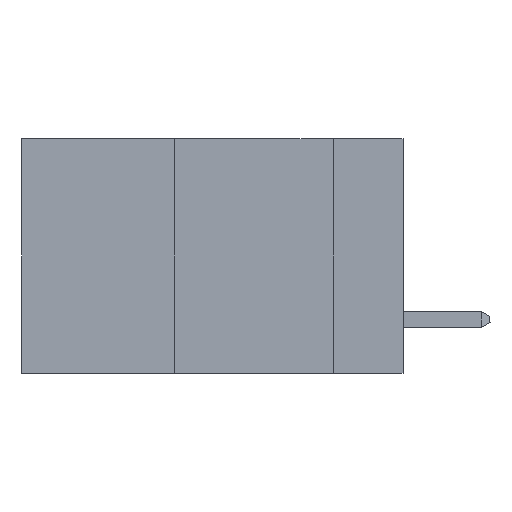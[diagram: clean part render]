
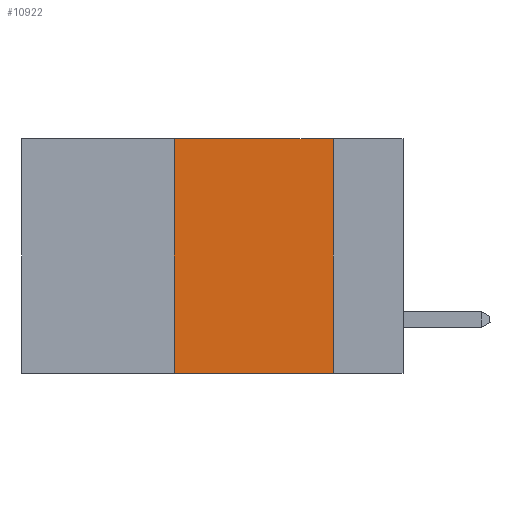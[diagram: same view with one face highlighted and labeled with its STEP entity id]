
A CAD part, left-side view. The second image highlights one B-rep face of the part: STEP entity #10922.
In plain terms, the highlighted planar face has unit normal (-1, 0, 0).
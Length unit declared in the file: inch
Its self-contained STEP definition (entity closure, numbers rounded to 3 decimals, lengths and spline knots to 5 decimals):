
#52 = VECTOR ( 'NONE', #11046, 39.37008 ) ;
#77 = ORIENTED_EDGE ( 'NONE', *, *, #9463, .F. ) ;
#2467 = EDGE_CURVE ( 'NONE', #17926, #2953, #6915, .T. ) ;
#2491 = AXIS2_PLACEMENT_3D ( 'NONE', #14686, #11143, #19555 ) ;
#2776 = CARTESIAN_POINT ( 'NONE',  ( 0., 0.11, 0. ) ) ;
#2953 = VERTEX_POINT ( 'NONE', #15706 ) ;
#3175 = DIRECTION ( 'NONE',  ( 0., 0., 1. ) ) ;
#3890 = LINE ( 'NONE', #8832, #15743 ) ;
#6676 = EDGE_LOOP ( 'NONE', ( #77, #9416, #6730, #10353 ) ) ;
#6730 = ORIENTED_EDGE ( 'NONE', *, *, #2467, .F. ) ;
#6915 = LINE ( 'NONE', #16023, #14667 ) ;
#7152 = CARTESIAN_POINT ( 'NONE',  ( 0., 0.36, -0.37 ) ) ;
#7319 = DIRECTION ( 'NONE',  ( 0., -1., 0. ) ) ;
#8322 = CARTESIAN_POINT ( 'NONE',  ( 0., 0.11, 0. ) ) ;
#8512 = LINE ( 'NONE', #2776, #52 ) ;
#8832 = CARTESIAN_POINT ( 'NONE',  ( 0., 0.6, 0. ) ) ;
#9317 = EDGE_CURVE ( 'NONE', #17926, #13791, #16044, .T. ) ;
#9416 = ORIENTED_EDGE ( 'NONE', *, *, #17530, .F. ) ;
#9463 = EDGE_CURVE ( 'NONE', #18415, #13791, #8512, .T. ) ;
#10353 = ORIENTED_EDGE ( 'NONE', *, *, #9317, .T. ) ;
#10922 = ADVANCED_FACE ( 'NONE', ( #17234 ), #11379, .F. ) ;
#11046 = DIRECTION ( 'NONE',  ( 0., 0., -1. ) ) ;
#11143 = DIRECTION ( 'NONE',  ( 1., 0., 0. ) ) ;
#11379 = PLANE ( 'NONE',  #2491 ) ;
#13791 = VERTEX_POINT ( 'NONE', #14308 ) ;
#14308 = CARTESIAN_POINT ( 'NONE',  ( 0., 0.11, -0.37 ) ) ;
#14667 = VECTOR ( 'NONE', #3175, 39.37008 ) ;
#14686 = CARTESIAN_POINT ( 'NONE',  ( 0., 0.6, 0. ) ) ;
#15706 = CARTESIAN_POINT ( 'NONE',  ( 0., 0.36, 0. ) ) ;
#15743 = VECTOR ( 'NONE', #7319, 39.37008 ) ;
#16023 = CARTESIAN_POINT ( 'NONE',  ( 0., 0.36, 0. ) ) ;
#16044 = LINE ( 'NONE', #20507, #19856 ) ;
#17234 = FACE_OUTER_BOUND ( 'NONE', #6676, .T. ) ;
#17530 = EDGE_CURVE ( 'NONE', #2953, #18415, #3890, .T. ) ;
#17694 = DIRECTION ( 'NONE',  ( 0., -1., 0. ) ) ;
#17926 = VERTEX_POINT ( 'NONE', #7152 ) ;
#18415 = VERTEX_POINT ( 'NONE', #8322 ) ;
#19555 = DIRECTION ( 'NONE',  ( 0., 0., -1. ) ) ;
#19856 = VECTOR ( 'NONE', #17694, 39.37008 ) ;
#20507 = CARTESIAN_POINT ( 'NONE',  ( 0., 0.6, -0.37 ) ) ;
